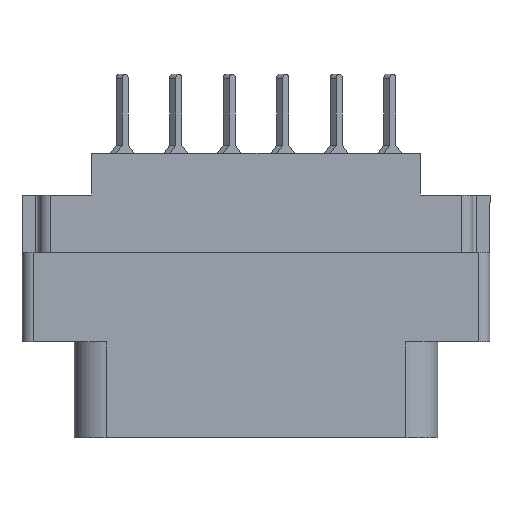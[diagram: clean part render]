
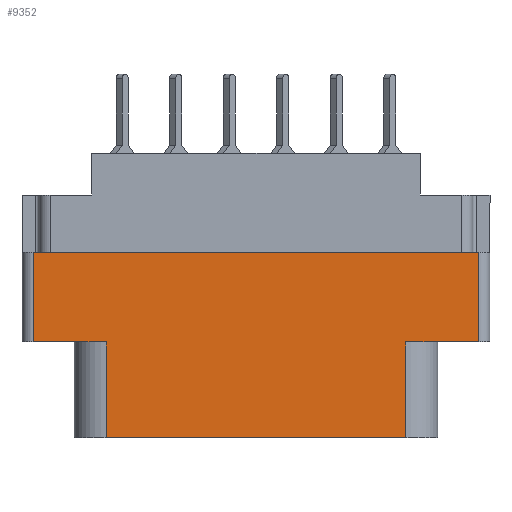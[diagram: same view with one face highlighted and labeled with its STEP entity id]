
A CAD part, front view. The second image highlights one B-rep face of the part: STEP entity #9352.
In plain terms, the highlighted planar face has unit normal (0, -1, 0).
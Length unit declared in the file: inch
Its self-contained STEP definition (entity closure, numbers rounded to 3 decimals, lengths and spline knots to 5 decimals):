
#196 = ORIENTED_EDGE ( 'NONE', *, *, #17530, .T. ) ;
#1904 = DIRECTION ( 'NONE',  ( 1., 0., 0. ) ) ;
#2563 = VECTOR ( 'NONE', #12477, 39.37008 ) ;
#2757 = CARTESIAN_POINT ( 'NONE',  ( 0.42, -0.343, -0.529 ) ) ;
#2942 = EDGE_CURVE ( 'NONE', #9389, #12229, #13379, .T. ) ;
#3553 = VERTEX_POINT ( 'NONE', #19786 ) ;
#3894 = LINE ( 'NONE', #4351, #15294 ) ;
#4050 = DIRECTION ( 'NONE',  ( 0., 0., -1. ) ) ;
#4252 = ORIENTED_EDGE ( 'NONE', *, *, #21302, .F. ) ;
#4351 = CARTESIAN_POINT ( 'NONE',  ( -0.656, -0.343, -0.277 ) ) ;
#4756 = VECTOR ( 'NONE', #4050, 39.37008 ) ;
#4791 = CARTESIAN_POINT ( 'NONE',  ( -0.42, -0.343, -0.529 ) ) ;
#4803 = DIRECTION ( 'NONE',  ( 1., 0., 0. ) ) ;
#4892 = AXIS2_PLACEMENT_3D ( 'NONE', #13472, #20981, #5694 ) ;
#5328 = VERTEX_POINT ( 'NONE', #16491 ) ;
#5361 = CARTESIAN_POINT ( 'NONE',  ( -0.624, -0.343, -0.277 ) ) ;
#5694 = DIRECTION ( 'NONE',  ( 0., 0., -1. ) ) ;
#6005 = CARTESIAN_POINT ( 'NONE',  ( -0.42, -0.343, -0.529 ) ) ;
#6837 = CARTESIAN_POINT ( 'NONE',  ( -0.624, -0.343, -0.798 ) ) ;
#7027 = ORIENTED_EDGE ( 'NONE', *, *, #13890, .F. ) ;
#7473 = VERTEX_POINT ( 'NONE', #11728 ) ;
#8094 = VECTOR ( 'NONE', #4803, 39.37008 ) ;
#8571 = LINE ( 'NONE', #6005, #4756 ) ;
#9352 = ADVANCED_FACE ( 'NONE', ( #14326 ), #13397, .T. ) ;
#9389 = VERTEX_POINT ( 'NONE', #20742 ) ;
#9474 = DIRECTION ( 'NONE',  ( -1., 0., 0. ) ) ;
#10045 = DIRECTION ( 'NONE',  ( 0., 0., 1. ) ) ;
#10144 = VERTEX_POINT ( 'NONE', #4791 ) ;
#10372 = CARTESIAN_POINT ( 'NONE',  ( 0.624, -0.343, -0.798 ) ) ;
#11280 = CARTESIAN_POINT ( 'NONE',  ( 0., -0.343, -0.529 ) ) ;
#11568 = ORIENTED_EDGE ( 'NONE', *, *, #21760, .T. ) ;
#11728 = CARTESIAN_POINT ( 'NONE',  ( 0.624, -0.343, -0.277 ) ) ;
#11852 = LINE ( 'NONE', #10372, #17648 ) ;
#12229 = VERTEX_POINT ( 'NONE', #13942 ) ;
#12280 = LINE ( 'NONE', #12848, #20454 ) ;
#12477 = DIRECTION ( 'NONE',  ( 0., 0., -1. ) ) ;
#12848 = CARTESIAN_POINT ( 'NONE',  ( 0., -0.343, -0.529 ) ) ;
#13379 = LINE ( 'NONE', #2757, #2563 ) ;
#13397 = PLANE ( 'NONE',  #4892 ) ;
#13472 = CARTESIAN_POINT ( 'NONE',  ( -0.624, -0.343, -0.798 ) ) ;
#13644 = LINE ( 'NONE', #14270, #8094 ) ;
#13748 = ORIENTED_EDGE ( 'NONE', *, *, #2942, .F. ) ;
#13890 = EDGE_CURVE ( 'NONE', #3553, #9389, #15828, .T. ) ;
#13942 = CARTESIAN_POINT ( 'NONE',  ( 0.42, -0.343, -0.798 ) ) ;
#14042 = VECTOR ( 'NONE', #16376, 39.37008 ) ;
#14270 = CARTESIAN_POINT ( 'NONE',  ( -0.624, -0.343, -0.798 ) ) ;
#14326 = FACE_OUTER_BOUND ( 'NONE', #14404, .T. ) ;
#14382 = EDGE_CURVE ( 'NONE', #18237, #20250, #21644, .T. ) ;
#14404 = EDGE_LOOP ( 'NONE', ( #11568, #196, #13748, #7027, #15242, #4252, #16840, #17878 ) ) ;
#15090 = EDGE_CURVE ( 'NONE', #18237, #10144, #12280, .T. ) ;
#15242 = ORIENTED_EDGE ( 'NONE', *, *, #18709, .T. ) ;
#15294 = VECTOR ( 'NONE', #23300, 39.37008 ) ;
#15828 = LINE ( 'NONE', #11280, #19354 ) ;
#16376 = DIRECTION ( 'NONE',  ( 0., 0., 1. ) ) ;
#16491 = CARTESIAN_POINT ( 'NONE',  ( -0.42, -0.343, -0.798 ) ) ;
#16598 = CARTESIAN_POINT ( 'NONE',  ( -0.624, -0.343, -0.529 ) ) ;
#16840 = ORIENTED_EDGE ( 'NONE', *, *, #14382, .F. ) ;
#17530 = EDGE_CURVE ( 'NONE', #5328, #12229, #13644, .T. ) ;
#17648 = VECTOR ( 'NONE', #10045, 39.37008 ) ;
#17878 = ORIENTED_EDGE ( 'NONE', *, *, #15090, .T. ) ;
#18237 = VERTEX_POINT ( 'NONE', #16598 ) ;
#18709 = EDGE_CURVE ( 'NONE', #3553, #7473, #11852, .T. ) ;
#19354 = VECTOR ( 'NONE', #9474, 39.37008 ) ;
#19786 = CARTESIAN_POINT ( 'NONE',  ( 0.624, -0.343, -0.529 ) ) ;
#20250 = VERTEX_POINT ( 'NONE', #5361 ) ;
#20454 = VECTOR ( 'NONE', #1904, 39.37008 ) ;
#20742 = CARTESIAN_POINT ( 'NONE',  ( 0.42, -0.343, -0.529 ) ) ;
#20981 = DIRECTION ( 'NONE',  ( 0., -1., 0. ) ) ;
#21302 = EDGE_CURVE ( 'NONE', #20250, #7473, #3894, .T. ) ;
#21644 = LINE ( 'NONE', #6837, #14042 ) ;
#21760 = EDGE_CURVE ( 'NONE', #10144, #5328, #8571, .T. ) ;
#23300 = DIRECTION ( 'NONE',  ( 1., 0., 0. ) ) ;
